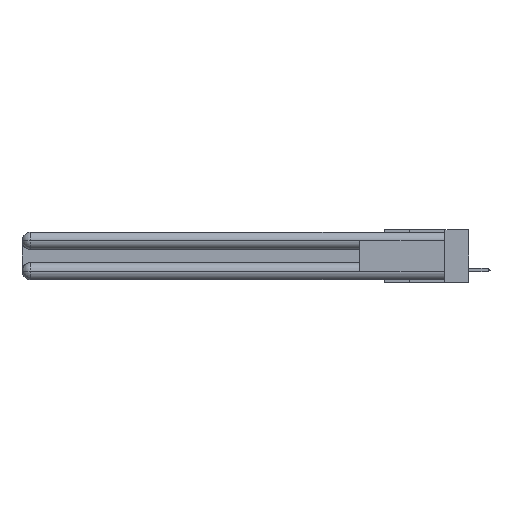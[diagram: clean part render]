
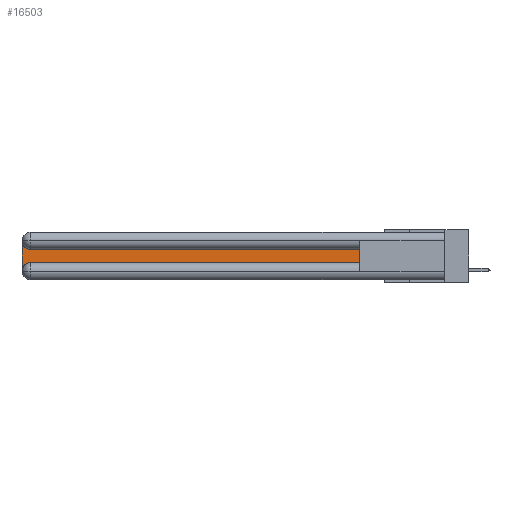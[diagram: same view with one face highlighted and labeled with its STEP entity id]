
A CAD part, left-side view. The second image highlights one B-rep face of the part: STEP entity #16503.
In plain terms, the highlighted planar face has unit normal (-1, 0, 0).
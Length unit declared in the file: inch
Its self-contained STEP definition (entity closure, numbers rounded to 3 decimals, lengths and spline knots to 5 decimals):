
#777 = CARTESIAN_POINT ( 'NONE',  ( 0.075, 2.94, -0.2175 ) ) ;
#1131 = DIRECTION ( 'NONE',  ( 0., 0., -1. ) ) ;
#1435 = LINE ( 'NONE', #18060, #7657 ) ;
#1935 = VERTEX_POINT ( 'NONE', #777 ) ;
#3166 = CARTESIAN_POINT ( 'NONE',  ( 0.075, 2.94, -0.0625 ) ) ;
#3726 = DIRECTION ( 'NONE',  ( 0., 0., -1. ) ) ;
#3825 = CARTESIAN_POINT ( 'NONE',  ( 0.075, 0.6, -0.2175 ) ) ;
#4679 = ORIENTED_EDGE ( 'NONE', *, *, #17014, .T. ) ;
#5587 = VERTEX_POINT ( 'NONE', #3825 ) ;
#6264 = VERTEX_POINT ( 'NONE', #7226 ) ;
#6356 = DIRECTION ( 'NONE',  ( 0., 1., 0. ) ) ;
#6571 = DIRECTION ( 'NONE',  ( 0., 0., 1. ) ) ;
#7226 = CARTESIAN_POINT ( 'NONE',  ( 0.075, 3., -0.0625 ) ) ;
#7657 = VECTOR ( 'NONE', #9504, 39.37008 ) ;
#7812 = DIRECTION ( 'NONE',  ( 0., 0., -1. ) ) ;
#8883 = AXIS2_PLACEMENT_3D ( 'NONE', #18028, #13577, #7812 ) ;
#9504 = DIRECTION ( 'NONE',  ( 0., 0., -1. ) ) ;
#10038 = CARTESIAN_POINT ( 'NONE',  ( 0.075, 0.6, -0.2175 ) ) ;
#10929 = CARTESIAN_POINT ( 'NONE',  ( 0.075, 0.6, -0.2175 ) ) ;
#11719 = ORIENTED_EDGE ( 'NONE', *, *, #20910, .T. ) ;
#11919 = LINE ( 'NONE', #10929, #18541 ) ;
#12087 = DIRECTION ( 'NONE',  ( 0., -1., 0. ) ) ;
#12859 = VERTEX_POINT ( 'NONE', #25387 ) ;
#13577 = DIRECTION ( 'NONE',  ( 1., 0., 0. ) ) ;
#14129 = PLANE ( 'NONE',  #17206 ) ;
#14215 = DIRECTION ( 'NONE',  ( 1., 0., 0. ) ) ;
#15176 = EDGE_CURVE ( 'NONE', #5587, #12859, #11919, .T. ) ;
#15527 = VERTEX_POINT ( 'NONE', #16411 ) ;
#15760 = CIRCLE ( 'NONE', #8883, 0.06 ) ;
#15778 = CARTESIAN_POINT ( 'NONE',  ( 0.075, 2.94, -0.1225 ) ) ;
#15875 = EDGE_LOOP ( 'NONE', ( #4679, #11719, #23538, #16443, #18834, #25117 ) ) ;
#16411 = CARTESIAN_POINT ( 'NONE',  ( 0.075, 3., -0.2775 ) ) ;
#16422 = FACE_OUTER_BOUND ( 'NONE', #15875, .T. ) ;
#16443 = ORIENTED_EDGE ( 'NONE', *, *, #17187, .T. ) ;
#16503 = ADVANCED_FACE ( 'NONE', ( #16422 ), #14129, .F. ) ;
#17014 = EDGE_CURVE ( 'NONE', #12859, #20477, #26313, .T. ) ;
#17088 = LINE ( 'NONE', #10038, #20039 ) ;
#17187 = EDGE_CURVE ( 'NONE', #15527, #1935, #15760, .T. ) ;
#17206 = AXIS2_PLACEMENT_3D ( 'NONE', #24402, #14215, #3726 ) ;
#17635 = EDGE_CURVE ( 'NONE', #1935, #5587, #17088, .T. ) ;
#17919 = DIRECTION ( 'NONE',  ( 1., 0., 0. ) ) ;
#18028 = CARTESIAN_POINT ( 'NONE',  ( 0.075, 2.94, -0.2775 ) ) ;
#18060 = CARTESIAN_POINT ( 'NONE',  ( 0.075, 3., -0.2175 ) ) ;
#18541 = VECTOR ( 'NONE', #6571, 39.37008 ) ;
#18807 = VECTOR ( 'NONE', #6356, 39.37008 ) ;
#18834 = ORIENTED_EDGE ( 'NONE', *, *, #17635, .T. ) ;
#20039 = VECTOR ( 'NONE', #12087, 39.37008 ) ;
#20477 = VERTEX_POINT ( 'NONE', #15778 ) ;
#20910 = EDGE_CURVE ( 'NONE', #20477, #6264, #26550, .T. ) ;
#21240 = AXIS2_PLACEMENT_3D ( 'NONE', #3166, #17919, #1131 ) ;
#23106 = EDGE_CURVE ( 'NONE', #6264, #15527, #1435, .T. ) ;
#23538 = ORIENTED_EDGE ( 'NONE', *, *, #23106, .T. ) ;
#24402 = CARTESIAN_POINT ( 'NONE',  ( 0.075, 3., -0.1225 ) ) ;
#25117 = ORIENTED_EDGE ( 'NONE', *, *, #15176, .T. ) ;
#25387 = CARTESIAN_POINT ( 'NONE',  ( 0.075, 0.6, -0.1225 ) ) ;
#26313 = LINE ( 'NONE', #27087, #18807 ) ;
#26550 = CIRCLE ( 'NONE', #21240, 0.06 ) ;
#27087 = CARTESIAN_POINT ( 'NONE',  ( 0.075, 0.6, -0.1225 ) ) ;
